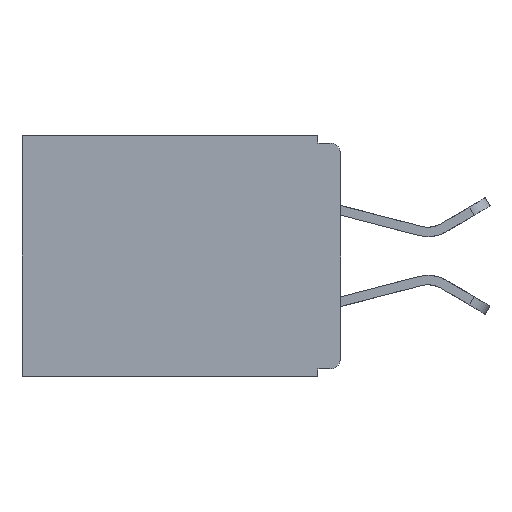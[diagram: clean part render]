
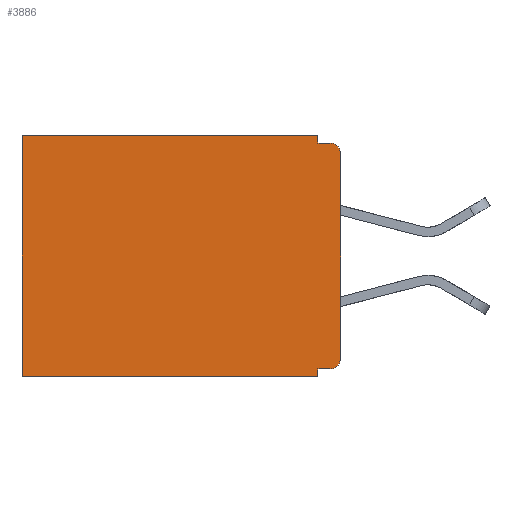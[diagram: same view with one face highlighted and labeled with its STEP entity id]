
A CAD part, left-side view. The second image highlights one B-rep face of the part: STEP entity #3886.
In plain terms, the highlighted planar face has unit normal (-1, 0, 0).
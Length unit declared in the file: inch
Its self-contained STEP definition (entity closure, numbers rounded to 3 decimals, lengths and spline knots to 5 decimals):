
#143 = CARTESIAN_POINT ( 'NONE',  ( 0.3, 0., -0.32 ) ) ;
#370 = CARTESIAN_POINT ( 'NONE',  ( 0.3, 0., -0.33 ) ) ;
#759 = LINE ( 'NONE', #23729, #24438 ) ;
#888 = CARTESIAN_POINT ( 'NONE',  ( 0.3, 0.015, -0.32 ) ) ;
#1840 = ORIENTED_EDGE ( 'NONE', *, *, #14202, .F. ) ;
#1888 = VECTOR ( 'NONE', #11842, 39.37008 ) ;
#2163 = ORIENTED_EDGE ( 'NONE', *, *, #8143, .T. ) ;
#2673 = CARTESIAN_POINT ( 'NONE',  ( 0.3, 0.031, 0. ) ) ;
#3125 = CARTESIAN_POINT ( 'NONE',  ( 0.3, 0.031, -0.33 ) ) ;
#3344 = ORIENTED_EDGE ( 'NONE', *, *, #13798, .T. ) ;
#3886 = ADVANCED_FACE ( 'NONE', ( #7040 ), #22103, .F. ) ;
#3972 = VECTOR ( 'NONE', #10503, 39.37008 ) ;
#5092 = DIRECTION ( 'NONE',  ( 0., 0., -1. ) ) ;
#6159 = EDGE_CURVE ( 'NONE', #18787, #6227, #16273, .T. ) ;
#6227 = VERTEX_POINT ( 'NONE', #3125 ) ;
#7040 = FACE_OUTER_BOUND ( 'NONE', #13966, .T. ) ;
#7192 = AXIS2_PLACEMENT_3D ( 'NONE', #8785, #24616, #11115 ) ;
#7798 = EDGE_CURVE ( 'NONE', #23311, #16727, #24557, .T. ) ;
#7856 = DIRECTION ( 'NONE',  ( 0., 0., -1. ) ) ;
#8129 = VECTOR ( 'NONE', #29073, 39.37008 ) ;
#8143 = EDGE_CURVE ( 'NONE', #11501, #16727, #26607, .T. ) ;
#8370 = CARTESIAN_POINT ( 'NONE',  ( 0.3, 0.015, -0.01 ) ) ;
#8508 = ORIENTED_EDGE ( 'NONE', *, *, #14638, .F. ) ;
#8785 = CARTESIAN_POINT ( 'NONE',  ( 0.3, 0.015, -0.305 ) ) ;
#9602 = EDGE_CURVE ( 'NONE', #19321, #24218, #28876, .T. ) ;
#9660 = DIRECTION ( 'NONE',  ( 1., 0., 0. ) ) ;
#10255 = ORIENTED_EDGE ( 'NONE', *, *, #6159, .F. ) ;
#10298 = VERTEX_POINT ( 'NONE', #8370 ) ;
#10503 = DIRECTION ( 'NONE',  ( 0., 0., -1. ) ) ;
#10517 = DIRECTION ( 'NONE',  ( 0., 0., -1. ) ) ;
#10891 = LINE ( 'NONE', #14165, #28748 ) ;
#11115 = DIRECTION ( 'NONE',  ( 0., 0., -1. ) ) ;
#11208 = CARTESIAN_POINT ( 'NONE',  ( 0.3, 0., -0.33 ) ) ;
#11501 = VERTEX_POINT ( 'NONE', #888 ) ;
#11697 = CARTESIAN_POINT ( 'NONE',  ( 0.3, 0., -0.33 ) ) ;
#11842 = DIRECTION ( 'NONE',  ( 0., 1., 0. ) ) ;
#12079 = ORIENTED_EDGE ( 'NONE', *, *, #7798, .F. ) ;
#12526 = CARTESIAN_POINT ( 'NONE',  ( 0.3, 0.031, -0.01 ) ) ;
#12601 = VECTOR ( 'NONE', #18902, 39.37008 ) ;
#12990 = VERTEX_POINT ( 'NONE', #14632 ) ;
#13320 = CARTESIAN_POINT ( 'NONE',  ( 0.3, 0.031, -0.33 ) ) ;
#13798 = EDGE_CURVE ( 'NONE', #19321, #12990, #16450, .T. ) ;
#13966 = EDGE_LOOP ( 'NONE', ( #12079, #17172, #16576, #15994, #3344, #15851, #8508, #10255, #1840, #2163 ) ) ;
#13974 = DIRECTION ( 'NONE',  ( -1., 0., 0. ) ) ;
#14165 = CARTESIAN_POINT ( 'NONE',  ( 0.3, 0., -0.01 ) ) ;
#14202 = EDGE_CURVE ( 'NONE', #11501, #18787, #15028, .T. ) ;
#14632 = CARTESIAN_POINT ( 'NONE',  ( 0.3, 0.437, 0. ) ) ;
#14638 = EDGE_CURVE ( 'NONE', #6227, #27449, #20254, .T. ) ;
#15028 = LINE ( 'NONE', #143, #1888 ) ;
#15091 = DIRECTION ( 'NONE',  ( 0., 1., 0. ) ) ;
#15851 = ORIENTED_EDGE ( 'NONE', *, *, #19585, .T. ) ;
#15994 = ORIENTED_EDGE ( 'NONE', *, *, #9602, .F. ) ;
#16273 = LINE ( 'NONE', #13320, #3972 ) ;
#16318 = EDGE_CURVE ( 'NONE', #24218, #10298, #10891, .T. ) ;
#16450 = LINE ( 'NONE', #26208, #19601 ) ;
#16576 = ORIENTED_EDGE ( 'NONE', *, *, #16318, .F. ) ;
#16727 = VERTEX_POINT ( 'NONE', #20048 ) ;
#17137 = VECTOR ( 'NONE', #5092, 39.37008 ) ;
#17172 = ORIENTED_EDGE ( 'NONE', *, *, #18048, .T. ) ;
#18048 = EDGE_CURVE ( 'NONE', #23311, #10298, #29020, .T. ) ;
#18469 = CARTESIAN_POINT ( 'NONE',  ( 0.3, 0.031, 0. ) ) ;
#18787 = VERTEX_POINT ( 'NONE', #27511 ) ;
#18902 = DIRECTION ( 'NONE',  ( 0., 0., -1. ) ) ;
#19321 = VERTEX_POINT ( 'NONE', #18469 ) ;
#19585 = EDGE_CURVE ( 'NONE', #12990, #27449, #759, .T. ) ;
#19601 = VECTOR ( 'NONE', #15091, 39.37008 ) ;
#20048 = CARTESIAN_POINT ( 'NONE',  ( 0.3, 0., -0.305 ) ) ;
#20254 = LINE ( 'NONE', #11208, #8129 ) ;
#20289 = AXIS2_PLACEMENT_3D ( 'NONE', #11697, #9660, #10517 ) ;
#22103 = PLANE ( 'NONE',  #20289 ) ;
#22989 = AXIS2_PLACEMENT_3D ( 'NONE', #27335, #13974, #29495 ) ;
#23111 = DIRECTION ( 'NONE',  ( 0., -1., 0. ) ) ;
#23311 = VERTEX_POINT ( 'NONE', #28383 ) ;
#23729 = CARTESIAN_POINT ( 'NONE',  ( 0.3, 0.437, -0.33 ) ) ;
#24218 = VERTEX_POINT ( 'NONE', #12526 ) ;
#24438 = VECTOR ( 'NONE', #7856, 39.37008 ) ;
#24557 = LINE ( 'NONE', #370, #12601 ) ;
#24616 = DIRECTION ( 'NONE',  ( -1., 0., 0. ) ) ;
#26208 = CARTESIAN_POINT ( 'NONE',  ( 0.3, 0., 0. ) ) ;
#26607 = CIRCLE ( 'NONE', #7192, 0.015 ) ;
#27335 = CARTESIAN_POINT ( 'NONE',  ( 0.3, 0.015, -0.025 ) ) ;
#27449 = VERTEX_POINT ( 'NONE', #29150 ) ;
#27511 = CARTESIAN_POINT ( 'NONE',  ( 0.3, 0.031, -0.32 ) ) ;
#28383 = CARTESIAN_POINT ( 'NONE',  ( 0.3, 0., -0.025 ) ) ;
#28748 = VECTOR ( 'NONE', #23111, 39.37008 ) ;
#28876 = LINE ( 'NONE', #2673, #17137 ) ;
#29020 = CIRCLE ( 'NONE', #22989, 0.015 ) ;
#29073 = DIRECTION ( 'NONE',  ( 0., 1., 0. ) ) ;
#29150 = CARTESIAN_POINT ( 'NONE',  ( 0.3, 0.437, -0.33 ) ) ;
#29495 = DIRECTION ( 'NONE',  ( 0., 0., -1. ) ) ;
